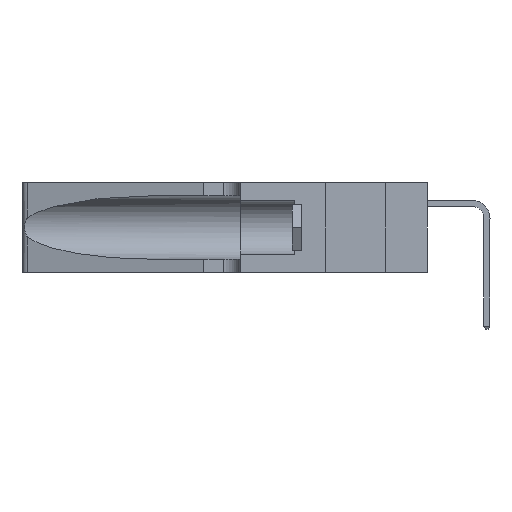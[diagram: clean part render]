
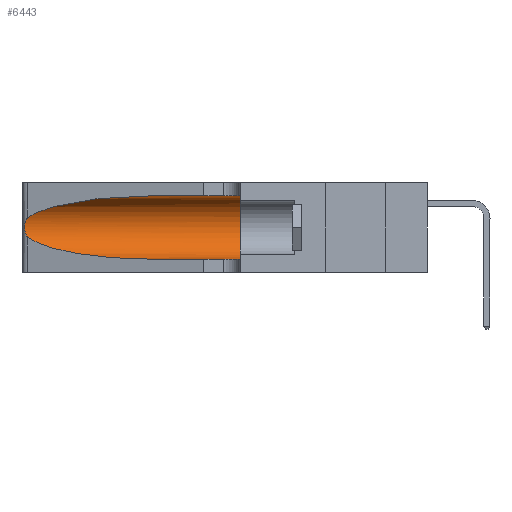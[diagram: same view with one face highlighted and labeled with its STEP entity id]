
A CAD part, left-side view. The second image highlights one B-rep face of the part: STEP entity #6443.
In plain terms, the highlighted cylindrical face has radius 3.308 mm (diameter 6.617 mm), a partial arc.
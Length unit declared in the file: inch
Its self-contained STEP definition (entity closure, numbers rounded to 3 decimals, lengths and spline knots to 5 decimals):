
#1378 = CARTESIAN_POINT ( 'NONE',  ( 0.25487, 1.22718, 0.22369 ) ) ;
#1385 = EDGE_CURVE ( 'NONE', #36486, #2738, #12993, .T. ) ;
#1572 = CARTESIAN_POINT ( 'NONE',  ( 0.25487, 1.22718, 0.22369 ) ) ;
#2738 = VERTEX_POINT ( 'NONE', #12314 ) ;
#2811 = ORIENTED_EDGE ( 'NONE', *, *, #12735, .T. ) ;
#2999 = EDGE_CURVE ( 'NONE', #36916, #36125, #38199, .T. ) ;
#3207 = CYLINDRICAL_SURFACE ( 'NONE', #24940, 0.13025 ) ;
#3485 = ORIENTED_EDGE ( 'NONE', *, *, #33556, .T. ) ;
#3833 =( BOUNDED_CURVE ( )  B_SPLINE_CURVE ( 3, ( #19115, #10284, #19247, #1378 ),
 .UNSPECIFIED., .F., .F. ) 
 B_SPLINE_CURVE_WITH_KNOTS ( ( 4, 4 ),
 ( 1.5708, 2.84003 ),
 .UNSPECIFIED. ) 
 CURVE ( )  GEOMETRIC_REPRESENTATION_ITEM ( )  RATIONAL_B_SPLINE_CURVE ( ( 1., 0.87, 0.87, 1. ) ) 
 REPRESENTATION_ITEM ( '' )  );
#4121 = DIRECTION ( 'NONE',  ( 0., 1., 0. ) ) ;
#4132 = FACE_OUTER_BOUND ( 'NONE', #25145, .T. ) ;
#4567 = CARTESIAN_POINT ( 'NONE',  ( 0.25787, 1.23484, 0.2124 ) ) ;
#4779 = LINE ( 'NONE', #21626, #27610 ) ;
#4821 = CARTESIAN_POINT ( 'NONE',  ( 0.25487, 1.22718, 0.14631 ) ) ;
#5202 = AXIS2_PLACEMENT_3D ( 'NONE', #21982, #4121, #24969 ) ;
#6443 = ADVANCED_FACE ( 'NONE', ( #4132 ), #3207, .F. ) ;
#7629 = CARTESIAN_POINT ( 'NONE',  ( 0.26018, 1.23835, 0.19895 ) ) ;
#9129 = VERTEX_POINT ( 'NONE', #30463 ) ;
#10284 = CARTESIAN_POINT ( 'NONE',  ( 0.18966, 0.96281, 0.31525 ) ) ;
#10578 = DIRECTION ( 'NONE',  ( 0., 0., -1. ) ) ;
#10600 = CARTESIAN_POINT ( 'NONE',  ( 0.26075, 1.23896, 0.178 ) ) ;
#11539 = ORIENTED_EDGE ( 'NONE', *, *, #1385, .F. ) ;
#12314 = CARTESIAN_POINT ( 'NONE',  ( 0.1305, 0.35, 0.31525 ) ) ;
#12595 = CARTESIAN_POINT ( 'NONE',  ( 0.25487, 1.22718, 0.22369 ) ) ;
#12735 = EDGE_CURVE ( 'NONE', #36486, #36916, #3833, .T. ) ;
#12993 = LINE ( 'NONE', #31592, #28780 ) ;
#13589 = CARTESIAN_POINT ( 'NONE',  ( 0.1305, 1.61858, 0.185 ) ) ;
#13616 = CARTESIAN_POINT ( 'NONE',  ( 0.25856, 1.23593, 0.16098 ) ) ;
#13846 = CARTESIAN_POINT ( 'NONE',  ( 0.18966, 0.96281, 0.05475 ) ) ;
#15065 = ORIENTED_EDGE ( 'NONE', *, *, #2999, .T. ) ;
#15801 = ORIENTED_EDGE ( 'NONE', *, *, #35945, .T. ) ;
#16070 = CIRCLE ( 'NONE', #5202, 0.13025 ) ;
#16603 = CARTESIAN_POINT ( 'NONE',  ( 0.25639, 1.23186, 0.15144 ) ) ;
#19115 = CARTESIAN_POINT ( 'NONE',  ( 0.1305, 0.72297, 0.31525 ) ) ;
#19247 = CARTESIAN_POINT ( 'NONE',  ( 0.2373, 1.15595, 0.28018 ) ) ;
#19430 = CARTESIAN_POINT ( 'NONE',  ( 0.25555, 1.22994, 0.2215 ) ) ;
#19564 = CARTESIAN_POINT ( 'NONE',  ( 0.25487, 1.22718, 0.14631 ) ) ;
#20678 = CARTESIAN_POINT ( 'NONE',  ( 0.25487, 1.22718, 0.14631 ) ) ;
#21626 = CARTESIAN_POINT ( 'NONE',  ( 0.1305, 1.61858, 0.05475 ) ) ;
#21982 = CARTESIAN_POINT ( 'NONE',  ( 0.1305, 0.35, 0.185 ) ) ;
#22009 = EDGE_CURVE ( 'NONE', #2738, #33252, #16070, .T. ) ;
#22427 = CARTESIAN_POINT ( 'NONE',  ( 0.25639, 1.23184, 0.21858 ) ) ;
#24143 = ORIENTED_EDGE ( 'NONE', *, *, #22009, .F. ) ;
#24940 = AXIS2_PLACEMENT_3D ( 'NONE', #13589, #34292, #10578 ) ;
#24969 = DIRECTION ( 'NONE',  ( 0., 0., 1. ) ) ;
#25145 = EDGE_LOOP ( 'NONE', ( #2811, #15065, #15801, #3485, #24143, #11539 ) ) ;
#25225 = CARTESIAN_POINT ( 'NONE',  ( 0.1305, 0.72297, 0.31525 ) ) ;
#25417 = CARTESIAN_POINT ( 'NONE',  ( 0.25854, 1.2359, 0.20912 ) ) ;
#27472 = DIRECTION ( 'NONE',  ( 0., -1., 0. ) ) ;
#27610 = VECTOR ( 'NONE', #27472, 39.37008 ) ;
#28399 = CARTESIAN_POINT ( 'NONE',  ( 0.26075, 1.23896, 0.19203 ) ) ;
#28632 = CARTESIAN_POINT ( 'NONE',  ( 0.2373, 1.15595, 0.08982 ) ) ;
#28780 = VECTOR ( 'NONE', #37894, 39.37008 ) ;
#30463 = CARTESIAN_POINT ( 'NONE',  ( 0.1305, 0.72297, 0.05475 ) ) ;
#31335 = CARTESIAN_POINT ( 'NONE',  ( 0.26017, 1.23833, 0.17102 ) ) ;
#31592 = CARTESIAN_POINT ( 'NONE',  ( 0.1305, 1.61858, 0.31525 ) ) ;
#32638 =( BOUNDED_CURVE ( )  B_SPLINE_CURVE ( 3, ( #4821, #28632, #13846, #34550 ),
 .UNSPECIFIED., .F., .F. ) 
 B_SPLINE_CURVE_WITH_KNOTS ( ( 4, 4 ),
 ( 3.44316, 4.71239 ),
 .UNSPECIFIED. ) 
 CURVE ( )  GEOMETRIC_REPRESENTATION_ITEM ( )  RATIONAL_B_SPLINE_CURVE ( ( 1., 0.87, 0.87, 1. ) ) 
 REPRESENTATION_ITEM ( '' )  );
#33252 = VERTEX_POINT ( 'NONE', #35064 ) ;
#33556 = EDGE_CURVE ( 'NONE', #9129, #33252, #4779, .T. ) ;
#34292 = DIRECTION ( 'NONE',  ( 0., -1., 0. ) ) ;
#34314 = CARTESIAN_POINT ( 'NONE',  ( 0.25789, 1.23486, 0.15765 ) ) ;
#34550 = CARTESIAN_POINT ( 'NONE',  ( 0.1305, 0.72297, 0.05475 ) ) ;
#35064 = CARTESIAN_POINT ( 'NONE',  ( 0.1305, 0.35, 0.05475 ) ) ;
#35945 = EDGE_CURVE ( 'NONE', #36125, #9129, #32638, .T. ) ;
#36125 = VERTEX_POINT ( 'NONE', #20678 ) ;
#36486 = VERTEX_POINT ( 'NONE', #25225 ) ;
#36916 = VERTEX_POINT ( 'NONE', #12595 ) ;
#37176 = CARTESIAN_POINT ( 'NONE',  ( 0.25555, 1.22993, 0.14849 ) ) ;
#37894 = DIRECTION ( 'NONE',  ( 0., -1., 0. ) ) ;
#38199 = B_SPLINE_CURVE_WITH_KNOTS ( 'NONE', 3,
 ( #1572, #19430, #22427, #4567, #25417, #7629, #28399, #10600, #31335, #13616, #34314, #16603, #37176, #19564 ),
 .UNSPECIFIED., .F., .F.,
 ( 4, 2, 2, 2, 2, 2, 4 ),
 ( 0., 0.00027, 0.00053, 0.00107, 0.0016, 0.00187, 0.00214 ),
 .UNSPECIFIED. ) ;
